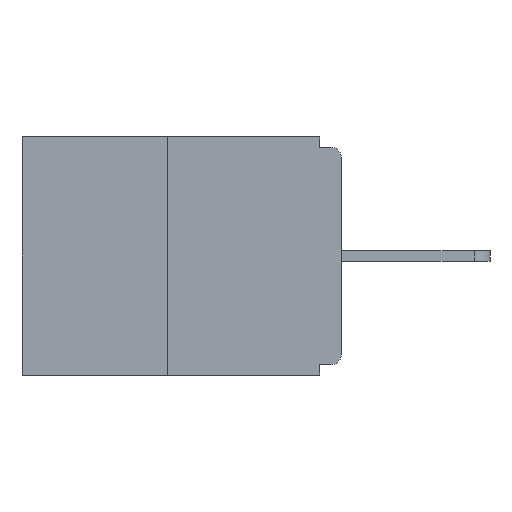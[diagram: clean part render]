
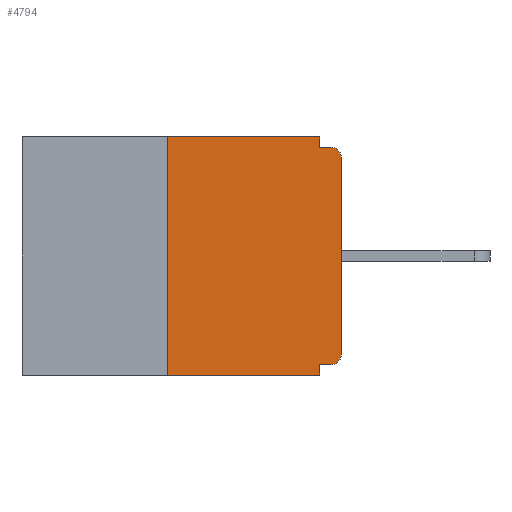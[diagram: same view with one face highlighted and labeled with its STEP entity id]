
A CAD part, left-side view. The second image highlights one B-rep face of the part: STEP entity #4794.
In plain terms, the highlighted planar face has unit normal (-1, 0, 0).
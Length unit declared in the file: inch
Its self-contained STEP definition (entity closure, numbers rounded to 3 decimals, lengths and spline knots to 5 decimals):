
#123 = CARTESIAN_POINT ( 'NONE',  ( 0., 0.25, 0. ) ) ;
#324 = CARTESIAN_POINT ( 'NONE',  ( 0., 0.015, -0.015 ) ) ;
#602 = EDGE_CURVE ( 'NONE', #4022, #17768, #1150, .T. ) ;
#983 = EDGE_CURVE ( 'NONE', #20627, #7261, #9475, .T. ) ;
#1006 = CARTESIAN_POINT ( 'NONE',  ( 0., 0.015, -0.03 ) ) ;
#1150 = LINE ( 'NONE', #7758, #4064 ) ;
#1234 = DIRECTION ( 'NONE',  ( -1., 0., 0. ) ) ;
#1244 = DIRECTION ( 'NONE',  ( 0., 0., -1. ) ) ;
#1288 = LINE ( 'NONE', #12539, #18810 ) ;
#1425 = DIRECTION ( 'NONE',  ( 0., 0., 1. ) ) ;
#1555 = CARTESIAN_POINT ( 'NONE',  ( 0., 0., -0.015 ) ) ;
#1998 = DIRECTION ( 'NONE',  ( 0., 0., -1. ) ) ;
#2295 = CARTESIAN_POINT ( 'NONE',  ( 0., 0.015, -0.313 ) ) ;
#2451 = ORIENTED_EDGE ( 'NONE', *, *, #602, .F. ) ;
#2569 = LINE ( 'NONE', #10046, #10610 ) ;
#2851 = AXIS2_PLACEMENT_3D ( 'NONE', #3915, #19167, #19146 ) ;
#3287 = VECTOR ( 'NONE', #1425, 39.37008 ) ;
#3661 = CARTESIAN_POINT ( 'NONE',  ( 0., 0.25, -0.343 ) ) ;
#3708 = EDGE_LOOP ( 'NONE', ( #21170, #3771, #8309, #8853, #13432, #18390, #5920, #19414, #19911, #2451 ) ) ;
#3771 = ORIENTED_EDGE ( 'NONE', *, *, #14374, .F. ) ;
#3915 = CARTESIAN_POINT ( 'NONE',  ( 0., 0.46, 0. ) ) ;
#4004 = CARTESIAN_POINT ( 'NONE',  ( 0., 0.46, -0.343 ) ) ;
#4022 = VERTEX_POINT ( 'NONE', #13548 ) ;
#4064 = VECTOR ( 'NONE', #5031, 39.37008 ) ;
#4466 = FACE_OUTER_BOUND ( 'NONE', #3708, .T. ) ;
#4794 = ADVANCED_FACE ( 'NONE', ( #4466 ), #9870, .F. ) ;
#5031 = DIRECTION ( 'NONE',  ( 0., 0., -1. ) ) ;
#5153 = EDGE_CURVE ( 'NONE', #20151, #8416, #14654, .T. ) ;
#5349 = CARTESIAN_POINT ( 'NONE',  ( 0., 0.031, -0.343 ) ) ;
#5350 = AXIS2_PLACEMENT_3D ( 'NONE', #1006, #1234, #1244 ) ;
#5392 = CARTESIAN_POINT ( 'NONE',  ( 0., 0.015, -0.328 ) ) ;
#5409 = EDGE_CURVE ( 'NONE', #15415, #8227, #10128, .T. ) ;
#5530 = VECTOR ( 'NONE', #1998, 39.37008 ) ;
#5547 = DIRECTION ( 'NONE',  ( 0., 1., 0. ) ) ;
#5615 = EDGE_CURVE ( 'NONE', #10739, #4022, #1288, .T. ) ;
#5920 = ORIENTED_EDGE ( 'NONE', *, *, #6714, .T. ) ;
#6714 = EDGE_CURVE ( 'NONE', #8227, #20627, #2569, .T. ) ;
#7025 = CARTESIAN_POINT ( 'NONE',  ( 0., 0.031, -0.015 ) ) ;
#7130 = LINE ( 'NONE', #1555, #15685 ) ;
#7213 = CARTESIAN_POINT ( 'NONE',  ( 0., 0.031, -0.328 ) ) ;
#7261 = VERTEX_POINT ( 'NONE', #324 ) ;
#7758 = CARTESIAN_POINT ( 'NONE',  ( 0., 0.031, 0. ) ) ;
#8227 = VERTEX_POINT ( 'NONE', #18434 ) ;
#8309 = ORIENTED_EDGE ( 'NONE', *, *, #10906, .T. ) ;
#8416 = VERTEX_POINT ( 'NONE', #5349 ) ;
#8853 = ORIENTED_EDGE ( 'NONE', *, *, #5153, .F. ) ;
#8901 = VECTOR ( 'NONE', #20894, 39.37008 ) ;
#9292 = DIRECTION ( 'NONE',  ( 0., 0., 1. ) ) ;
#9475 = CIRCLE ( 'NONE', #5350, 0.015 ) ;
#9870 = PLANE ( 'NONE',  #2851 ) ;
#10046 = CARTESIAN_POINT ( 'NONE',  ( 0., 0., 0. ) ) ;
#10128 = CIRCLE ( 'NONE', #16851, 0.015 ) ;
#10229 = VECTOR ( 'NONE', #5547, 39.37008 ) ;
#10610 = VECTOR ( 'NONE', #9292, 39.37008 ) ;
#10739 = VERTEX_POINT ( 'NONE', #123 ) ;
#10764 = LINE ( 'NONE', #12382, #10229 ) ;
#10906 = EDGE_CURVE ( 'NONE', #12095, #8416, #13484, .T. ) ;
#11540 = EDGE_CURVE ( 'NONE', #15415, #20151, #10764, .T. ) ;
#11675 = CARTESIAN_POINT ( 'NONE',  ( 0., 0.25, 0. ) ) ;
#11795 = DIRECTION ( 'NONE',  ( 0., -1., 0. ) ) ;
#12095 = VERTEX_POINT ( 'NONE', #3661 ) ;
#12296 = DIRECTION ( 'NONE',  ( 0., 0., -1. ) ) ;
#12382 = CARTESIAN_POINT ( 'NONE',  ( 0., 0., -0.328 ) ) ;
#12489 = DIRECTION ( 'NONE',  ( -1., 0., 0. ) ) ;
#12539 = CARTESIAN_POINT ( 'NONE',  ( 0., 0.46, 0. ) ) ;
#13432 = ORIENTED_EDGE ( 'NONE', *, *, #11540, .F. ) ;
#13484 = LINE ( 'NONE', #4004, #8901 ) ;
#13548 = CARTESIAN_POINT ( 'NONE',  ( 0., 0.031, 0. ) ) ;
#14374 = EDGE_CURVE ( 'NONE', #12095, #10739, #16375, .T. ) ;
#14654 = LINE ( 'NONE', #15830, #5530 ) ;
#14980 = DIRECTION ( 'NONE',  ( 0., -1., 0. ) ) ;
#15415 = VERTEX_POINT ( 'NONE', #5392 ) ;
#15685 = VECTOR ( 'NONE', #11795, 39.37008 ) ;
#15830 = CARTESIAN_POINT ( 'NONE',  ( 0., 0.031, -0.343 ) ) ;
#16375 = LINE ( 'NONE', #11675, #3287 ) ;
#16851 = AXIS2_PLACEMENT_3D ( 'NONE', #2295, #12489, #12296 ) ;
#17768 = VERTEX_POINT ( 'NONE', #7025 ) ;
#18220 = EDGE_CURVE ( 'NONE', #17768, #7261, #7130, .T. ) ;
#18390 = ORIENTED_EDGE ( 'NONE', *, *, #5409, .T. ) ;
#18434 = CARTESIAN_POINT ( 'NONE',  ( 0., 0., -0.313 ) ) ;
#18732 = CARTESIAN_POINT ( 'NONE',  ( 0., 0., -0.03 ) ) ;
#18810 = VECTOR ( 'NONE', #14980, 39.37008 ) ;
#19146 = DIRECTION ( 'NONE',  ( 0., 0., -1. ) ) ;
#19167 = DIRECTION ( 'NONE',  ( 1., 0., 0. ) ) ;
#19414 = ORIENTED_EDGE ( 'NONE', *, *, #983, .T. ) ;
#19911 = ORIENTED_EDGE ( 'NONE', *, *, #18220, .F. ) ;
#20151 = VERTEX_POINT ( 'NONE', #7213 ) ;
#20627 = VERTEX_POINT ( 'NONE', #18732 ) ;
#20894 = DIRECTION ( 'NONE',  ( 0., -1., 0. ) ) ;
#21170 = ORIENTED_EDGE ( 'NONE', *, *, #5615, .F. ) ;
